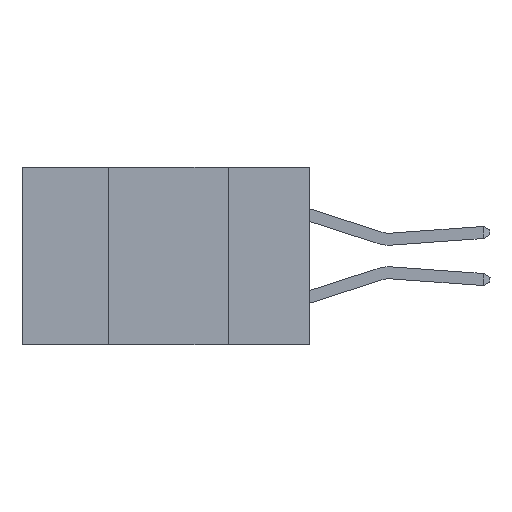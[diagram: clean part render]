
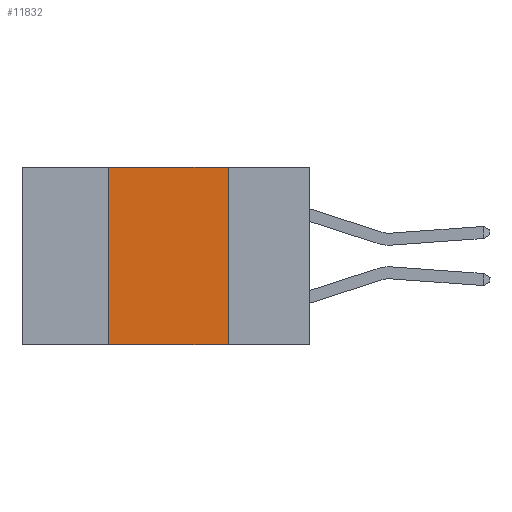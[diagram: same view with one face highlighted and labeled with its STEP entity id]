
A CAD part, left-side view. The second image highlights one B-rep face of the part: STEP entity #11832.
In plain terms, the highlighted planar face has unit normal (-1, 0, 0).
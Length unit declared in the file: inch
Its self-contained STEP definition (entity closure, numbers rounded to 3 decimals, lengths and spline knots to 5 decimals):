
#3285 = ORIENTED_EDGE ( 'NONE', *, *, #8604, .F. ) ;
#3415 = VECTOR ( 'NONE', #16409, 39.37008 ) ;
#4159 = VERTEX_POINT ( 'NONE', #6066 ) ;
#4223 = LINE ( 'NONE', #28782, #3415 ) ;
#4443 = VERTEX_POINT ( 'NONE', #17448 ) ;
#4693 = ORIENTED_EDGE ( 'NONE', *, *, #8763, .F. ) ;
#6066 = CARTESIAN_POINT ( 'NONE',  ( 0., 0.42, -0.37 ) ) ;
#6334 = DIRECTION ( 'NONE',  ( 1., 0., 0. ) ) ;
#6552 = VECTOR ( 'NONE', #9369, 39.37008 ) ;
#6993 = CARTESIAN_POINT ( 'NONE',  ( 0., 0.17, -0.37 ) ) ;
#7013 = EDGE_CURVE ( 'NONE', #4159, #10486, #4223, .T. ) ;
#8604 = EDGE_CURVE ( 'NONE', #10908, #10486, #22709, .T. ) ;
#8763 = EDGE_CURVE ( 'NONE', #4443, #10908, #14629, .T. ) ;
#9369 = DIRECTION ( 'NONE',  ( 0., 0., -1. ) ) ;
#10486 = VERTEX_POINT ( 'NONE', #6993 ) ;
#10908 = VERTEX_POINT ( 'NONE', #13709 ) ;
#11039 = DIRECTION ( 'NONE',  ( 0., 0., -1. ) ) ;
#11832 = ADVANCED_FACE ( 'NONE', ( #20908 ), #23904, .F. ) ;
#13088 = ORIENTED_EDGE ( 'NONE', *, *, #19584, .F. ) ;
#13709 = CARTESIAN_POINT ( 'NONE',  ( 0., 0.17, 0. ) ) ;
#14629 = LINE ( 'NONE', #14827, #30354 ) ;
#14827 = CARTESIAN_POINT ( 'NONE',  ( 0., 0.6, 0. ) ) ;
#15629 = ORIENTED_EDGE ( 'NONE', *, *, #7013, .T. ) ;
#16409 = DIRECTION ( 'NONE',  ( 0., -1., 0. ) ) ;
#16999 = AXIS2_PLACEMENT_3D ( 'NONE', #31809, #6334, #11039 ) ;
#17448 = CARTESIAN_POINT ( 'NONE',  ( 0., 0.42, 0. ) ) ;
#17470 = LINE ( 'NONE', #25538, #33156 ) ;
#19584 = EDGE_CURVE ( 'NONE', #4159, #4443, #17470, .T. ) ;
#20908 = FACE_OUTER_BOUND ( 'NONE', #23387, .T. ) ;
#22709 = LINE ( 'NONE', #24272, #6552 ) ;
#23387 = EDGE_LOOP ( 'NONE', ( #3285, #4693, #13088, #15629 ) ) ;
#23904 = PLANE ( 'NONE',  #16999 ) ;
#24272 = CARTESIAN_POINT ( 'NONE',  ( 0., 0.17, 0. ) ) ;
#25310 = DIRECTION ( 'NONE',  ( 0., 0., 1. ) ) ;
#25313 = DIRECTION ( 'NONE',  ( 0., -1., 0. ) ) ;
#25538 = CARTESIAN_POINT ( 'NONE',  ( 0., 0.42, 0. ) ) ;
#28782 = CARTESIAN_POINT ( 'NONE',  ( 0., 0.6, -0.37 ) ) ;
#30354 = VECTOR ( 'NONE', #25313, 39.37008 ) ;
#31809 = CARTESIAN_POINT ( 'NONE',  ( 0., 0.6, 0. ) ) ;
#33156 = VECTOR ( 'NONE', #25310, 39.37008 ) ;
